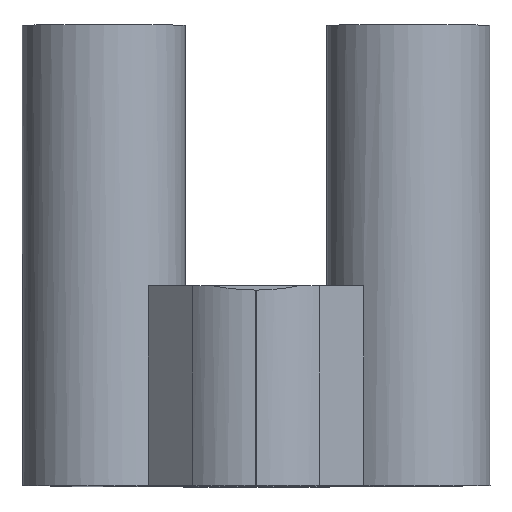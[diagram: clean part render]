
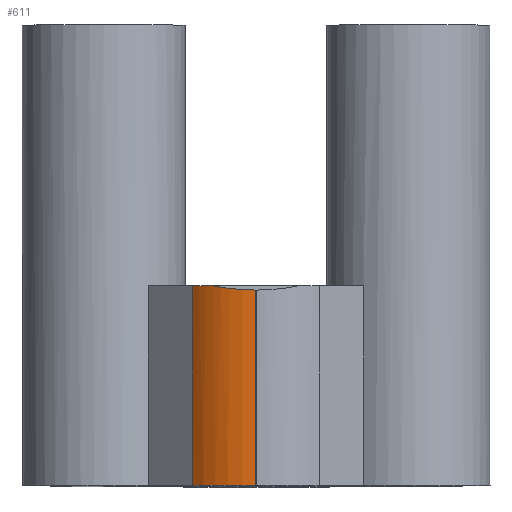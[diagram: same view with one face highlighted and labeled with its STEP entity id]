
A CAD part, top view. The second image highlights one B-rep face of the part: STEP entity #611.
In plain terms, the highlighted cylindrical face has radius 12 mm (diameter 24 mm), a partial arc.
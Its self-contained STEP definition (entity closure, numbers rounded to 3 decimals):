
#22 = VERTEX_POINT('',#23);
#23 = CARTESIAN_POINT('',(-5.857,-223.172,
    39.607));
#32 = PLANE('',#33);
#33 = AXIS2_PLACEMENT_3D('',#34,#35,#36);
#34 = CARTESIAN_POINT('',(-12.45,-207.21,
    -0.619));
#35 = DIRECTION('',(0.,0.93,0.369)
  );
#36 = DIRECTION('',(0.,-0.369,0.93)
  );
#43 = PLANE('',#44);
#44 = AXIS2_PLACEMENT_3D('',#45,#46,#47);
#45 = CARTESIAN_POINT('',(-91.608,-223.151,-26.394
    ));
#46 = DIRECTION('',(0.,-1.,
    0.));
#47 = DIRECTION('',(0.,0.,-1.));
#54 = EDGE_CURVE('',#55,#22,#57,.T.);
#55 = VERTEX_POINT('',#56);
#56 = CARTESIAN_POINT('',(-0.029,-223.771,
    41.117));
#57 = SURFACE_CURVE('',#58,(#63,#74),.PCURVE_S1.);
#58 = ELLIPSE('',#59,12.909,12.);
#59 = AXIS2_PLACEMENT_3D('',#60,#61,#62);
#60 = CARTESIAN_POINT('',(-0.029,-219.01,
    29.118));
#61 = DIRECTION('',(0.,-0.93,-0.369)
  );
#62 = DIRECTION('',(0.,0.369,-0.93)
  );
#63 = PCURVE('',#32,#64);
#64 = DEFINITIONAL_REPRESENTATION('',(#65),#73);
#65 = ( BOUNDED_CURVE() B_SPLINE_CURVE(2,(#66,#67,#68,#69,#70,#71,#72),
.UNSPECIFIED.,.F.,.F.) B_SPLINE_CURVE_WITH_KNOTS((1,2,2,2,2,1),(
    -2.094,0.,2.094,4.189,6.283,
8.378),.UNSPECIFIED.) CURVE() GEOMETRIC_REPRESENTATION_ITEM() 
RATIONAL_B_SPLINE_CURVE((1.,0.5,1.,0.5,1.,0.5,1.)) REPRESENTATION_ITEM(
  '') );
#66 = CARTESIAN_POINT('',(19.085,12.421));
#67 = CARTESIAN_POINT('',(19.085,33.205));
#68 = CARTESIAN_POINT('',(38.448,22.813));
#69 = CARTESIAN_POINT('',(57.81,12.421));
#70 = CARTESIAN_POINT('',(38.448,2.028));
#71 = CARTESIAN_POINT('',(19.085,-8.364));
#72 = CARTESIAN_POINT('',(19.085,12.421));
#73 = ( GEOMETRIC_REPRESENTATION_CONTEXT(2) 
PARAMETRIC_REPRESENTATION_CONTEXT() REPRESENTATION_CONTEXT('2D SPACE',''
  ) );
#74 = PCURVE('',#75,#80);
#75 = CYLINDRICAL_SURFACE('',#76,12.);
#76 = AXIS2_PLACEMENT_3D('',#77,#78,#79);
#77 = CARTESIAN_POINT('',(-0.029,-250.068,
    29.109));
#78 = DIRECTION('',(0.,1.,
    0.));
#79 = DIRECTION('',(0.,0.,
    1.));
#80 = DEFINITIONAL_REPRESENTATION('',(#81),#91);
#81 = B_SPLINE_CURVE_WITH_KNOTS('',8,(#82,#83,#84,#85,#86,#87,#88,#89,
    #90),.UNSPECIFIED.,.F.,.F.,(9,9),(3.142,3.649),
  .PIECEWISE_BEZIER_KNOTS.);
#82 = CARTESIAN_POINT('',(0.,26.301));
#83 = CARTESIAN_POINT('',(-0.063,26.301));
#84 = CARTESIAN_POINT('',(-0.127,26.323));
#85 = CARTESIAN_POINT('',(-0.19,26.367));
#86 = CARTESIAN_POINT('',(-0.254,26.432));
#87 = CARTESIAN_POINT('',(-0.317,26.519));
#88 = CARTESIAN_POINT('',(-0.38,26.626));
#89 = CARTESIAN_POINT('',(-0.444,26.754));
#90 = CARTESIAN_POINT('',(-0.507,26.9));
#91 = ( GEOMETRIC_REPRESENTATION_CONTEXT(2) 
PARAMETRIC_REPRESENTATION_CONTEXT() REPRESENTATION_CONTEXT('2D SPACE',''
  ) );
#109 = PLANE('',#110);
#110 = AXIS2_PLACEMENT_3D('',#111,#112,#113);
#111 = CARTESIAN_POINT('',(6.2,-223.072,
    41.117));
#112 = DIRECTION('',(0.,0.,
    1.));
#113 = DIRECTION('',(-1.,0.,0.));
#162 = EDGE_CURVE('',#22,#163,#165,.T.);
#163 = VERTEX_POINT('',#164);
#164 = CARTESIAN_POINT('',(-8.515,-223.171,
    37.602));
#165 = SURFACE_CURVE('',#166,(#171,#178),.PCURVE_S1.);
#166 = CIRCLE('',#167,12.);
#167 = AXIS2_PLACEMENT_3D('',#168,#169,#170);
#168 = CARTESIAN_POINT('',(-0.029,-223.168,
    29.117));
#169 = DIRECTION('',(0.,-1.,
    0.));
#170 = DIRECTION('',(0.,0.,1.));
#171 = PCURVE('',#43,#172);
#172 = DEFINITIONAL_REPRESENTATION('',(#173),#177);
#173 = CIRCLE('',#174,12.);
#174 = AXIS2_PLACEMENT_2D('',#175,#176);
#175 = CARTESIAN_POINT('',(-55.511,91.579));
#176 = DIRECTION('',(-1.,0.));
#177 = ( GEOMETRIC_REPRESENTATION_CONTEXT(2) 
PARAMETRIC_REPRESENTATION_CONTEXT() REPRESENTATION_CONTEXT('2D SPACE',''
  ) );
#178 = PCURVE('',#75,#179);
#179 = DEFINITIONAL_REPRESENTATION('',(#180),#184);
#180 = LINE('',#181,#182);
#181 = CARTESIAN_POINT('',(0.,26.9));
#182 = VECTOR('',#183,1.);
#183 = DIRECTION('',(-1.,0.));
#184 = ( GEOMETRIC_REPRESENTATION_CONTEXT(2) 
PARAMETRIC_REPRESENTATION_CONTEXT() REPRESENTATION_CONTEXT('2D SPACE',''
  ) );
#201 = PLANE('',#202);
#202 = AXIS2_PLACEMENT_3D('',#203,#204,#205);
#203 = CARTESIAN_POINT('',(-5.61,-223.072,
    40.507));
#204 = DIRECTION('',(0.707,0.,-0.707)
  );
#205 = DIRECTION('',(-0.707,0.,-0.707
    ));
#611 = ADVANCED_FACE('',(#612),#75,.T.);
#612 = FACE_BOUND('',#613,.F.);
#613 = EDGE_LOOP('',(#614,#615,#638,#671,#692));
#614 = ORIENTED_EDGE('',*,*,#54,.F.);
#615 = ORIENTED_EDGE('',*,*,#616,.F.);
#616 = EDGE_CURVE('',#617,#55,#619,.T.);
#617 = VERTEX_POINT('',#618);
#618 = CARTESIAN_POINT('',(-0.029,-250.072,
    41.109));
#619 = SURFACE_CURVE('',#620,(#624,#631),.PCURVE_S1.);
#620 = LINE('',#621,#622);
#621 = CARTESIAN_POINT('',(-0.029,-250.072,
    41.109));
#622 = VECTOR('',#623,1.);
#623 = DIRECTION('',(0.,1.,
    0.));
#624 = PCURVE('',#75,#625);
#625 = DEFINITIONAL_REPRESENTATION('',(#626),#630);
#626 = LINE('',#627,#628);
#627 = CARTESIAN_POINT('',(0.,0.));
#628 = VECTOR('',#629,1.);
#629 = DIRECTION('',(0.,1.));
#630 = ( GEOMETRIC_REPRESENTATION_CONTEXT(2) 
PARAMETRIC_REPRESENTATION_CONTEXT() REPRESENTATION_CONTEXT('2D SPACE',''
  ) );
#631 = PCURVE('',#109,#632);
#632 = DEFINITIONAL_REPRESENTATION('',(#633),#637);
#633 = LINE('',#634,#635);
#634 = CARTESIAN_POINT('',(6.229,27.));
#635 = VECTOR('',#636,1.);
#636 = DIRECTION('',(0.,-1.));
#637 = ( GEOMETRIC_REPRESENTATION_CONTEXT(2) 
PARAMETRIC_REPRESENTATION_CONTEXT() REPRESENTATION_CONTEXT('2D SPACE',''
  ) );
#638 = ORIENTED_EDGE('',*,*,#639,.T.);
#639 = EDGE_CURVE('',#617,#640,#642,.T.);
#640 = VERTEX_POINT('',#641);
#641 = CARTESIAN_POINT('',(-8.515,-250.071,
    37.594));
#642 = SURFACE_CURVE('',#643,(#648,#655),.PCURVE_S1.);
#643 = CIRCLE('',#644,12.);
#644 = AXIS2_PLACEMENT_3D('',#645,#646,#647);
#645 = CARTESIAN_POINT('',(-0.029,-250.068,
    29.109));
#646 = DIRECTION('',(0.,-1.,
    0.));
#647 = DIRECTION('',(0.,0.,1.));
#648 = PCURVE('',#75,#649);
#649 = DEFINITIONAL_REPRESENTATION('',(#650),#654);
#650 = LINE('',#651,#652);
#651 = CARTESIAN_POINT('',(0.,0.));
#652 = VECTOR('',#653,1.);
#653 = DIRECTION('',(-1.,0.));
#654 = ( GEOMETRIC_REPRESENTATION_CONTEXT(2) 
PARAMETRIC_REPRESENTATION_CONTEXT() REPRESENTATION_CONTEXT('2D SPACE',''
  ) );
#655 = PCURVE('',#656,#661);
#656 = PLANE('',#657);
#657 = AXIS2_PLACEMENT_3D('',#658,#659,#660);
#658 = CARTESIAN_POINT('',(80.558,-250.049,
    -34.746));
#659 = DIRECTION('',(0.,1.,
    0.));
#660 = DIRECTION('',(0.,0.,
    1.));
#661 = DEFINITIONAL_REPRESENTATION('',(#662),#670);
#662 = ( BOUNDED_CURVE() B_SPLINE_CURVE(2,(#663,#664,#665,#666,#667,#668
,#669),.UNSPECIFIED.,.T.,.F.) B_SPLINE_CURVE_WITH_KNOTS((1,2,2,2,2,1),(
    -2.094,0.,2.094,4.189,6.283,
8.378),.UNSPECIFIED.) CURVE() GEOMETRIC_REPRESENTATION_ITEM() 
RATIONAL_B_SPLINE_CURVE((1.,0.5,1.,0.5,1.,0.5,1.)) REPRESENTATION_ITEM(
  '') );
#663 = CARTESIAN_POINT('',(75.855,-80.587));
#664 = CARTESIAN_POINT('',(75.855,-101.372));
#665 = CARTESIAN_POINT('',(57.855,-90.979));
#666 = CARTESIAN_POINT('',(39.855,-80.587));
#667 = CARTESIAN_POINT('',(57.855,-70.195));
#668 = CARTESIAN_POINT('',(75.855,-59.803));
#669 = CARTESIAN_POINT('',(75.855,-80.587));
#670 = ( GEOMETRIC_REPRESENTATION_CONTEXT(2) 
PARAMETRIC_REPRESENTATION_CONTEXT() REPRESENTATION_CONTEXT('2D SPACE',''
  ) );
#671 = ORIENTED_EDGE('',*,*,#672,.T.);
#672 = EDGE_CURVE('',#640,#163,#673,.T.);
#673 = SURFACE_CURVE('',#674,(#678,#685),.PCURVE_S1.);
#674 = LINE('',#675,#676);
#675 = CARTESIAN_POINT('',(-8.515,-250.071,
    37.594));
#676 = VECTOR('',#677,1.);
#677 = DIRECTION('',(0.,1.,
    0.));
#678 = PCURVE('',#75,#679);
#679 = DEFINITIONAL_REPRESENTATION('',(#680),#684);
#680 = LINE('',#681,#682);
#681 = CARTESIAN_POINT('',(-0.785,0.));
#682 = VECTOR('',#683,1.);
#683 = DIRECTION('',(0.,1.));
#684 = ( GEOMETRIC_REPRESENTATION_CONTEXT(2) 
PARAMETRIC_REPRESENTATION_CONTEXT() REPRESENTATION_CONTEXT('2D SPACE',''
  ) );
#685 = PCURVE('',#201,#686);
#686 = DEFINITIONAL_REPRESENTATION('',(#687),#691);
#687 = LINE('',#688,#689);
#688 = CARTESIAN_POINT('',(4.108,-27.));
#689 = VECTOR('',#690,1.);
#690 = DIRECTION('',(0.,1.));
#691 = ( GEOMETRIC_REPRESENTATION_CONTEXT(2) 
PARAMETRIC_REPRESENTATION_CONTEXT() REPRESENTATION_CONTEXT('2D SPACE',''
  ) );
#692 = ORIENTED_EDGE('',*,*,#162,.F.);
